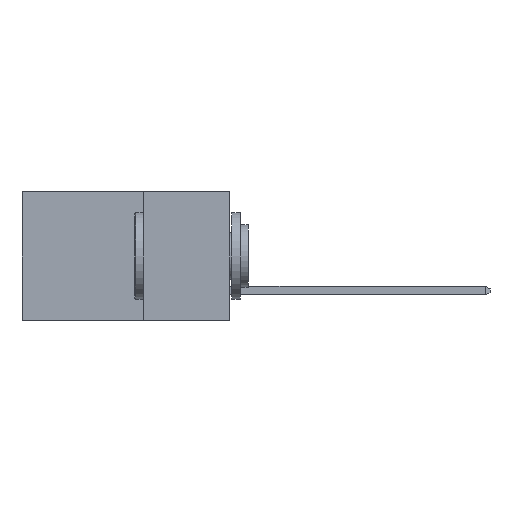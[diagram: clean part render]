
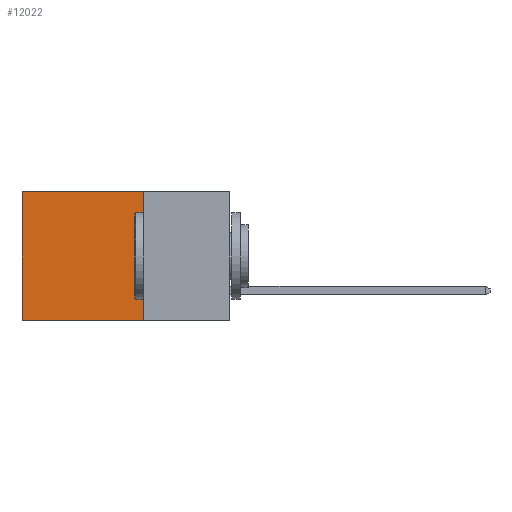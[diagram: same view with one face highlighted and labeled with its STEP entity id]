
A CAD part, left-side view. The second image highlights one B-rep face of the part: STEP entity #12022.
In plain terms, the highlighted planar face has unit normal (-1, 0, 0).
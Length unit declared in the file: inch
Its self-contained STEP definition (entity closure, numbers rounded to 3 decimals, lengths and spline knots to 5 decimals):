
#76 = CARTESIAN_POINT ( 'NONE',  ( 0.2615, 0.25, -0.37 ) ) ;
#115 = VERTEX_POINT ( 'NONE', #1199 ) ;
#328 = EDGE_CURVE ( 'NONE', #14248, #115, #7645, .T. ) ;
#689 = CARTESIAN_POINT ( 'NONE',  ( 0.2615, 0.25, -0.37 ) ) ;
#1103 = VECTOR ( 'NONE', #14225, 39.37008 ) ;
#1199 = CARTESIAN_POINT ( 'NONE',  ( 0.2615, 0.6, -0.37 ) ) ;
#1498 = LINE ( 'NONE', #2858, #12574 ) ;
#2858 = CARTESIAN_POINT ( 'NONE',  ( 0.2615, 0.25, 0. ) ) ;
#3999 = DIRECTION ( 'NONE',  ( 0., 1., 0. ) ) ;
#4473 = DIRECTION ( 'NONE',  ( 1., 0., 0. ) ) ;
#5185 = EDGE_CURVE ( 'NONE', #7888, #14006, #1498, .T. ) ;
#5612 = CARTESIAN_POINT ( 'NONE',  ( 0.2615, 0.25, -0.37 ) ) ;
#5755 = AXIS2_PLACEMENT_3D ( 'NONE', #5612, #4473, #9010 ) ;
#5796 = FACE_OUTER_BOUND ( 'NONE', #6255, .T. ) ;
#6255 = EDGE_LOOP ( 'NONE', ( #13740, #11303, #8018, #12406 ) ) ;
#6292 = EDGE_CURVE ( 'NONE', #14006, #115, #7138, .T. ) ;
#6764 = VECTOR ( 'NONE', #9576, 39.37008 ) ;
#7051 = DIRECTION ( 'NONE',  ( 0., 1., 0. ) ) ;
#7138 = LINE ( 'NONE', #8524, #6764 ) ;
#7645 = LINE ( 'NONE', #12941, #8187 ) ;
#7814 = CARTESIAN_POINT ( 'NONE',  ( 0.2615, 0.25, 0. ) ) ;
#7888 = VERTEX_POINT ( 'NONE', #7814 ) ;
#8018 = ORIENTED_EDGE ( 'NONE', *, *, #8610, .F. ) ;
#8187 = VECTOR ( 'NONE', #3999, 39.37008 ) ;
#8524 = CARTESIAN_POINT ( 'NONE',  ( 0.2615, 0.6, -0.37 ) ) ;
#8539 = LINE ( 'NONE', #689, #1103 ) ;
#8610 = EDGE_CURVE ( 'NONE', #7888, #14248, #8539, .T. ) ;
#9010 = DIRECTION ( 'NONE',  ( 0., 0., -1. ) ) ;
#9576 = DIRECTION ( 'NONE',  ( 0., 0., -1. ) ) ;
#9643 = CARTESIAN_POINT ( 'NONE',  ( 0.2615, 0.6, 0. ) ) ;
#11151 = PLANE ( 'NONE',  #5755 ) ;
#11303 = ORIENTED_EDGE ( 'NONE', *, *, #328, .F. ) ;
#12022 = ADVANCED_FACE ( 'NONE', ( #5796 ), #11151, .F. ) ;
#12406 = ORIENTED_EDGE ( 'NONE', *, *, #5185, .T. ) ;
#12574 = VECTOR ( 'NONE', #7051, 39.37008 ) ;
#12941 = CARTESIAN_POINT ( 'NONE',  ( 0.2615, 0.25, -0.37 ) ) ;
#13740 = ORIENTED_EDGE ( 'NONE', *, *, #6292, .T. ) ;
#14006 = VERTEX_POINT ( 'NONE', #9643 ) ;
#14225 = DIRECTION ( 'NONE',  ( 0., 0., -1. ) ) ;
#14248 = VERTEX_POINT ( 'NONE', #76 ) ;
